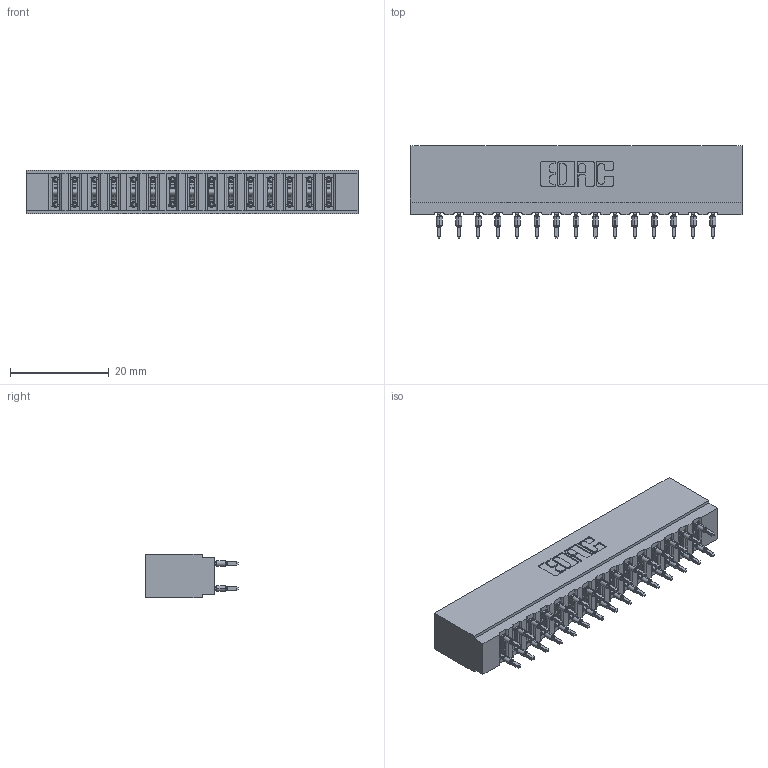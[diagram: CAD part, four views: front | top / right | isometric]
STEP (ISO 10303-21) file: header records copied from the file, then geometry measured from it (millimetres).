
FILE_DESCRIPTION (( 'STEP AP203' ), '1' );
FILE_NAME ('717-030-560-201.STEP', '2026-02-20T17:34:38', ( '' ), ( '' ), 'SwSTEP 2.0', 'SolidWorks 2023', '' );
FILE_SCHEMA (( 'CONFIG_CONTROL_DESIGN' ));
Length unit declared in the file: millimetre
Products named in the file (3): 717 Part_Insulator Option - 06; 717-030-560-201; 745-292-001_560
Assembly tree (31 placements, depth 2):
  717-030-560-201
    717 Part_Insulator Option - 06
    745-292-001_560  x30
Bounding box: 67.31 x 18.78 x 8.89 mm (x, y, z)
Volume: 6054.9 mm3; surface area: 9427.7 mm2
Topology: 31 solids, 31 shells, 3064 faces, 8381 edges, 5326 vertices
Faces by surface type: plane 1599, cylinder 685, bspline 600, torus 180
Entity records: 29688 total; most frequent: CARTESIAN_POINT 5665, ORIENTED_EDGE 5046, DIRECTION 4435, EDGE_CURVE 2523, VECTOR 2243, LINE 2243, VERTEX_POINT 1614, AXIS2_PLACEMENT_3D 1096
